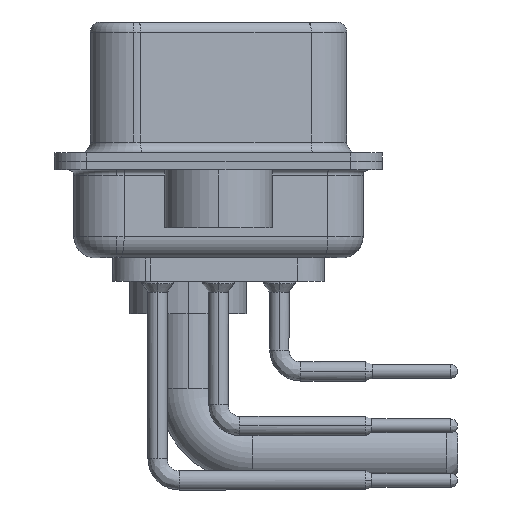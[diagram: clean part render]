
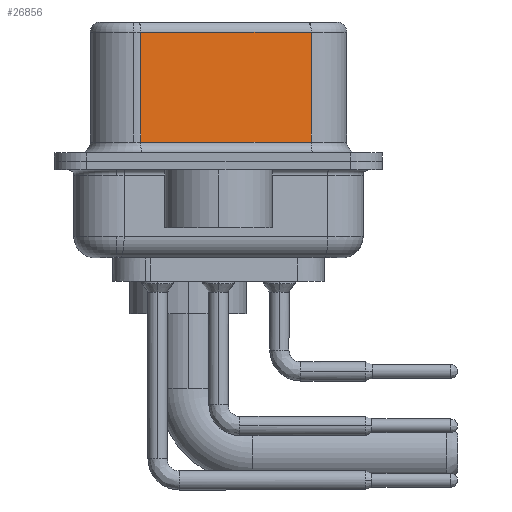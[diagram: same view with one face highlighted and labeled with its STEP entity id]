
A CAD part, left-side view. The second image highlights one B-rep face of the part: STEP entity #26856.
In plain terms, the highlighted planar face has unit normal (-0.985, -0.174, 0).
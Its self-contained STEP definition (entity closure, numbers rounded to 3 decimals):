
#4257 = VERTEX_POINT ( 'NONE', #32936 ) ;
#4289 = LINE ( 'NONE', #15505, #24794 ) ;
#4301 = CARTESIAN_POINT ( 'NONE',  ( 3.73, 3.628, 0.9 ) ) ;
#5842 = DIRECTION ( 'NONE',  ( -0.174, 0.985, 0. ) ) ;
#7091 = ORIENTED_EDGE ( 'NONE', *, *, #32947, .T. ) ;
#7923 = VERTEX_POINT ( 'NONE', #31751 ) ;
#8471 = FACE_OUTER_BOUND ( 'NONE', #22446, .T. ) ;
#8770 = LINE ( 'NONE', #25463, #16013 ) ;
#9497 = LINE ( 'NONE', #17946, #34672 ) ;
#11776 = LINE ( 'NONE', #22973, #25964 ) ;
#12354 = ORIENTED_EDGE ( 'NONE', *, *, #18201, .T. ) ;
#14168 = ORIENTED_EDGE ( 'NONE', *, *, #31139, .F. ) ;
#14352 = DIRECTION ( 'NONE',  ( -0.174, 0.985, 0. ) ) ;
#15505 = CARTESIAN_POINT ( 'NONE',  ( 5.132, -4.322, 0.9 ) ) ;
#15730 = ORIENTED_EDGE ( 'NONE', *, *, #33390, .T. ) ;
#15748 = DIRECTION ( 'NONE',  ( 0., 0., -1. ) ) ;
#16013 = VECTOR ( 'NONE', #5842, 1000. ) ;
#16940 = AXIS2_PLACEMENT_3D ( 'NONE', #27738, #28283, #14352 ) ;
#17946 = CARTESIAN_POINT ( 'NONE',  ( 5.132, -4.322, 6.52 ) ) ;
#18201 = EDGE_CURVE ( 'NONE', #4257, #7923, #8770, .T. ) ;
#19669 = PLANE ( 'NONE',  #16940 ) ;
#22446 = EDGE_LOOP ( 'NONE', ( #14168, #12354, #15730, #7091 ) ) ;
#22973 = CARTESIAN_POINT ( 'NONE',  ( 3.73, 3.628, 6.52 ) ) ;
#24092 = VERTEX_POINT ( 'NONE', #35903 ) ;
#24794 = VECTOR ( 'NONE', #29956, 1000. ) ;
#25463 = CARTESIAN_POINT ( 'NONE',  ( 5.132, -4.322, 6.02 ) ) ;
#25964 = VECTOR ( 'NONE', #34153, 1000. ) ;
#26856 = ADVANCED_FACE ( 'NONE', ( #8471 ), #19669, .F. ) ;
#27738 = CARTESIAN_POINT ( 'NONE',  ( 5.132, -4.322, 6.52 ) ) ;
#28283 = DIRECTION ( 'NONE',  ( 0.985, 0.174, 0. ) ) ;
#29956 = DIRECTION ( 'NONE',  ( 0.174, -0.985, 0. ) ) ;
#31139 = EDGE_CURVE ( 'NONE', #4257, #24092, #9497, .T. ) ;
#31751 = CARTESIAN_POINT ( 'NONE',  ( 3.73, 3.628, 6.02 ) ) ;
#32936 = CARTESIAN_POINT ( 'NONE',  ( 5.132, -4.322, 6.02 ) ) ;
#32947 = EDGE_CURVE ( 'NONE', #36139, #24092, #4289, .T. ) ;
#33390 = EDGE_CURVE ( 'NONE', #7923, #36139, #11776, .T. ) ;
#34153 = DIRECTION ( 'NONE',  ( 0., 0., -1. ) ) ;
#34672 = VECTOR ( 'NONE', #15748, 1000. ) ;
#35903 = CARTESIAN_POINT ( 'NONE',  ( 5.132, -4.322, 0.9 ) ) ;
#36139 = VERTEX_POINT ( 'NONE', #4301 ) ;
